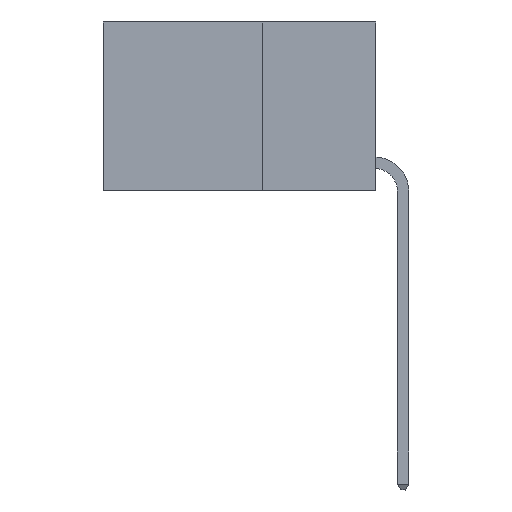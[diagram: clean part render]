
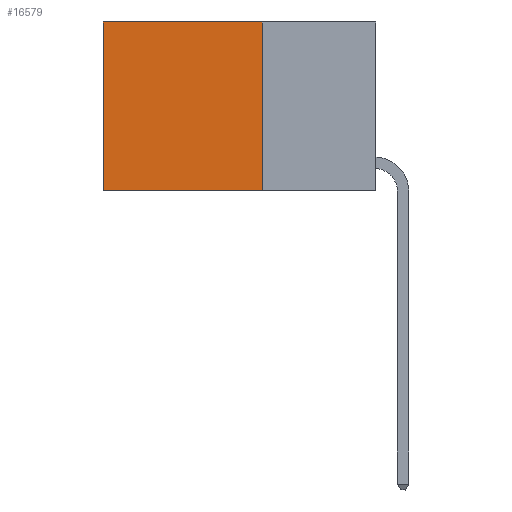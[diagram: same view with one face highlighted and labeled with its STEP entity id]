
A CAD part, left-side view. The second image highlights one B-rep face of the part: STEP entity #16579.
In plain terms, the highlighted planar face has unit normal (-1, 0, 0).
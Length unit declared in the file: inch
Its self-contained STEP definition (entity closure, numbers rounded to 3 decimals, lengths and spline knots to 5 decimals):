
#1147 = VERTEX_POINT ( 'NONE', #19844 ) ;
#1951 = CARTESIAN_POINT ( 'NONE',  ( 0.2625, 0.25, 0. ) ) ;
#2260 = VERTEX_POINT ( 'NONE', #7828 ) ;
#4099 = LINE ( 'NONE', #1951, #19413 ) ;
#4144 = DIRECTION ( 'NONE',  ( 0., 1., 0. ) ) ;
#6093 = VERTEX_POINT ( 'NONE', #26687 ) ;
#7063 = CARTESIAN_POINT ( 'NONE',  ( 0.2625, 0.6, 0. ) ) ;
#7828 = CARTESIAN_POINT ( 'NONE',  ( 0.2625, 0.6, 0. ) ) ;
#8054 = VECTOR ( 'NONE', #24980, 39.37008 ) ;
#8768 = EDGE_CURVE ( 'NONE', #1147, #9512, #14961, .T. ) ;
#8800 = DIRECTION ( 'NONE',  ( 0., 0., -1. ) ) ;
#9512 = VERTEX_POINT ( 'NONE', #23252 ) ;
#12200 = EDGE_CURVE ( 'NONE', #2260, #6093, #16920, .T. ) ;
#13599 = ORIENTED_EDGE ( 'NONE', *, *, #12200, .T. ) ;
#14408 = EDGE_LOOP ( 'NONE', ( #13599, #17402, #18342, #24364 ) ) ;
#14961 = LINE ( 'NONE', #24999, #25981 ) ;
#14974 = CARTESIAN_POINT ( 'NONE',  ( 0.2625, 0.25, 0. ) ) ;
#16579 = ADVANCED_FACE ( 'NONE', ( #17939 ), #17004, .F. ) ;
#16920 = LINE ( 'NONE', #7063, #19812 ) ;
#17004 = PLANE ( 'NONE',  #24692 ) ;
#17402 = ORIENTED_EDGE ( 'NONE', *, *, #26189, .F. ) ;
#17939 = FACE_OUTER_BOUND ( 'NONE', #14408, .T. ) ;
#18342 = ORIENTED_EDGE ( 'NONE', *, *, #8768, .F. ) ;
#19057 = LINE ( 'NONE', #22906, #8054 ) ;
#19413 = VECTOR ( 'NONE', #4144, 39.37008 ) ;
#19812 = VECTOR ( 'NONE', #23665, 39.37008 ) ;
#19844 = CARTESIAN_POINT ( 'NONE',  ( 0.2625, 0.25, 0. ) ) ;
#20862 = DIRECTION ( 'NONE',  ( 0., 0., -1. ) ) ;
#21163 = DIRECTION ( 'NONE',  ( 1., 0., 0. ) ) ;
#22906 = CARTESIAN_POINT ( 'NONE',  ( 0.2625, 0.25, -0.37 ) ) ;
#23252 = CARTESIAN_POINT ( 'NONE',  ( 0.2625, 0.25, -0.37 ) ) ;
#23665 = DIRECTION ( 'NONE',  ( 0., 0., -1. ) ) ;
#24364 = ORIENTED_EDGE ( 'NONE', *, *, #25503, .T. ) ;
#24692 = AXIS2_PLACEMENT_3D ( 'NONE', #14974, #21163, #8800 ) ;
#24980 = DIRECTION ( 'NONE',  ( 0., 1., 0. ) ) ;
#24999 = CARTESIAN_POINT ( 'NONE',  ( 0.2625, 0.25, 0. ) ) ;
#25503 = EDGE_CURVE ( 'NONE', #1147, #2260, #4099, .T. ) ;
#25981 = VECTOR ( 'NONE', #20862, 39.37008 ) ;
#26189 = EDGE_CURVE ( 'NONE', #9512, #6093, #19057, .T. ) ;
#26687 = CARTESIAN_POINT ( 'NONE',  ( 0.2625, 0.6, -0.37 ) ) ;
